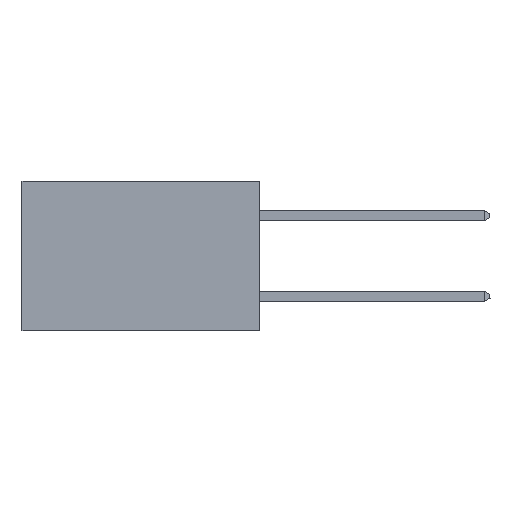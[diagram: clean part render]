
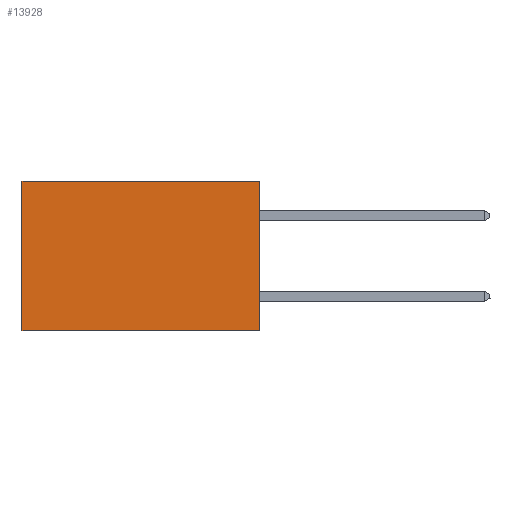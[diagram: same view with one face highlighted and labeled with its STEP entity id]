
A CAD part, left-side view. The second image highlights one B-rep face of the part: STEP entity #13928.
In plain terms, the highlighted planar face has unit normal (-1, 0, 0).
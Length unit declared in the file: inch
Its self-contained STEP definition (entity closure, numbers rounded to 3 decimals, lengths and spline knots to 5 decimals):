
#385 = DIRECTION ( 'NONE',  ( 0., 1., 0. ) ) ;
#1374 = VECTOR ( 'NONE', #16896, 39.37008 ) ;
#1742 = ORIENTED_EDGE ( 'NONE', *, *, #2101, .F. ) ;
#1985 = CARTESIAN_POINT ( 'NONE',  ( 0.277, 0., -0.37 ) ) ;
#1992 = LINE ( 'NONE', #20900, #1374 ) ;
#2101 = EDGE_CURVE ( 'NONE', #5679, #24782, #5016, .T. ) ;
#2501 = DIRECTION ( 'NONE',  ( 0., 0., -1. ) ) ;
#4246 = PLANE ( 'NONE',  #20117 ) ;
#4418 = VECTOR ( 'NONE', #385, 39.37008 ) ;
#5016 = LINE ( 'NONE', #1985, #4418 ) ;
#5077 = VECTOR ( 'NONE', #16838, 39.37008 ) ;
#5679 = VERTEX_POINT ( 'NONE', #18011 ) ;
#6183 = DIRECTION ( 'NONE',  ( 1., 0., 0. ) ) ;
#7540 = ORIENTED_EDGE ( 'NONE', *, *, #19724, .T. ) ;
#9223 = ORIENTED_EDGE ( 'NONE', *, *, #19557, .F. ) ;
#11846 = EDGE_LOOP ( 'NONE', ( #21954, #1742, #9223, #7540 ) ) ;
#11959 = LINE ( 'NONE', #23741, #22358 ) ;
#12606 = VERTEX_POINT ( 'NONE', #23110 ) ;
#13574 = CARTESIAN_POINT ( 'NONE',  ( 0.277, 0.59, 0. ) ) ;
#13928 = ADVANCED_FACE ( 'NONE', ( #22610 ), #4246, .F. ) ;
#14468 = VERTEX_POINT ( 'NONE', #13574 ) ;
#14886 = CARTESIAN_POINT ( 'NONE',  ( 0.277, 0., -0.37 ) ) ;
#15350 = LINE ( 'NONE', #14886, #5077 ) ;
#16838 = DIRECTION ( 'NONE',  ( 0., 0., -1. ) ) ;
#16896 = DIRECTION ( 'NONE',  ( 0., 1., 0. ) ) ;
#18011 = CARTESIAN_POINT ( 'NONE',  ( 0.277, 0., -0.37 ) ) ;
#18193 = CARTESIAN_POINT ( 'NONE',  ( 0.277, 0.59, -0.37 ) ) ;
#19557 = EDGE_CURVE ( 'NONE', #12606, #5679, #15350, .T. ) ;
#19715 = DIRECTION ( 'NONE',  ( 0., 0., -1. ) ) ;
#19724 = EDGE_CURVE ( 'NONE', #12606, #14468, #1992, .T. ) ;
#19955 = EDGE_CURVE ( 'NONE', #14468, #24782, #11959, .T. ) ;
#20117 = AXIS2_PLACEMENT_3D ( 'NONE', #23528, #6183, #19715 ) ;
#20900 = CARTESIAN_POINT ( 'NONE',  ( 0.277, 0., 0. ) ) ;
#21954 = ORIENTED_EDGE ( 'NONE', *, *, #19955, .T. ) ;
#22358 = VECTOR ( 'NONE', #2501, 39.37008 ) ;
#22610 = FACE_OUTER_BOUND ( 'NONE', #11846, .T. ) ;
#23110 = CARTESIAN_POINT ( 'NONE',  ( 0.277, 0., 0. ) ) ;
#23528 = CARTESIAN_POINT ( 'NONE',  ( 0.277, 0., -0.37 ) ) ;
#23741 = CARTESIAN_POINT ( 'NONE',  ( 0.277, 0.59, -0.37 ) ) ;
#24782 = VERTEX_POINT ( 'NONE', #18193 ) ;
